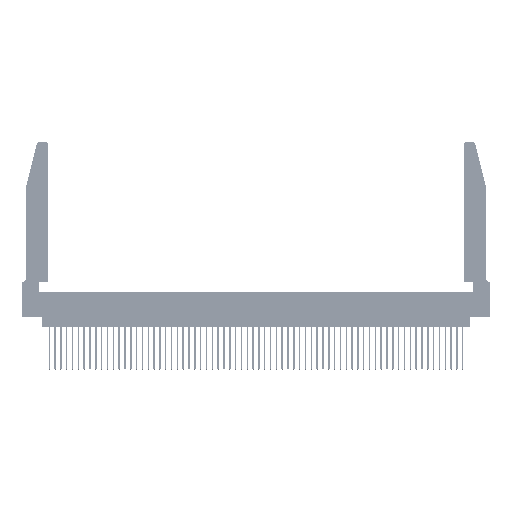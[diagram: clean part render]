
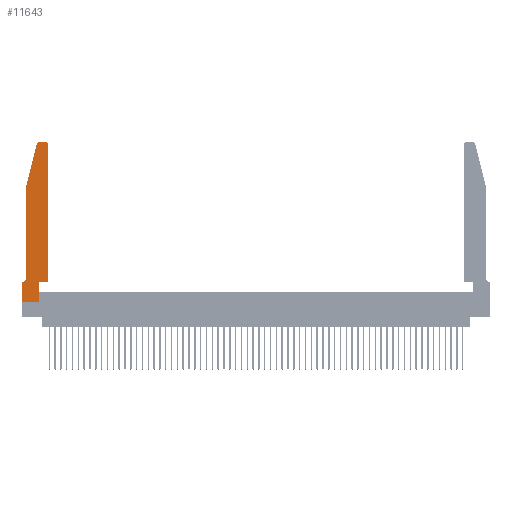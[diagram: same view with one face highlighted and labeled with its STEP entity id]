
A CAD part, top view. The second image highlights one B-rep face of the part: STEP entity #11643.
In plain terms, the highlighted planar face has unit normal (0, 0, 1).
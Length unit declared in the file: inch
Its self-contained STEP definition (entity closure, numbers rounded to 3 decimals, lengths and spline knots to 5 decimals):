
#1697 = CARTESIAN_POINT ( 'NONE',  ( 0.2865, 0., 0.37 ) ) ;
#2220 = CARTESIAN_POINT ( 'NONE',  ( 0.284, 2.72, 0.37 ) ) ;
#2479 = DIRECTION ( 'NONE',  ( 1., 0., 0. ) ) ;
#2614 = ORIENTED_EDGE ( 'NONE', *, *, #24294, .T. ) ;
#3371 = VERTEX_POINT ( 'NONE', #28870 ) ;
#3982 = VECTOR ( 'NONE', #50351, 39.37008 ) ;
#4497 = CARTESIAN_POINT ( 'NONE',  ( 0.2865, 0.35, 0.37 ) ) ;
#6109 = DIRECTION ( 'NONE',  ( 0., 0., -1. ) ) ;
#6855 = VERTEX_POINT ( 'NONE', #46864 ) ;
#7852 = ORIENTED_EDGE ( 'NONE', *, *, #39142, .T. ) ;
#8134 = CARTESIAN_POINT ( 'NONE',  ( 0.4205, 2.72, 0.37 ) ) ;
#8221 = VECTOR ( 'NONE', #50771, 39.37008 ) ;
#9159 = ORIENTED_EDGE ( 'NONE', *, *, #27788, .T. ) ;
#9622 = LINE ( 'NONE', #38343, #36553 ) ;
#9731 = CARTESIAN_POINT ( 'NONE',  ( 0.4205, 2.75, 0.37 ) ) ;
#10589 = DIRECTION ( 'NONE',  ( 1., 0., 0. ) ) ;
#10696 = VECTOR ( 'NONE', #14450, 39.37008 ) ;
#11239 = VERTEX_POINT ( 'NONE', #39124 ) ;
#11420 = VECTOR ( 'NONE', #52880, 39.37008 ) ;
#11643 = ADVANCED_FACE ( 'NONE', ( #20713 ), #40673, .T. ) ;
#12100 = VERTEX_POINT ( 'NONE', #16924 ) ;
#12194 = VERTEX_POINT ( 'NONE', #21421 ) ;
#12627 = DIRECTION ( 'NONE',  ( 1., 0., 0. ) ) ;
#14081 = CARTESIAN_POINT ( 'NONE',  ( 0., 0.35, 0.37 ) ) ;
#14450 = DIRECTION ( 'NONE',  ( 0., -1., 0. ) ) ;
#14970 = CARTESIAN_POINT ( 'NONE',  ( 0.0755, 0.35, 0.37 ) ) ;
#15146 = LINE ( 'NONE', #14970, #8221 ) ;
#16924 = CARTESIAN_POINT ( 'NONE',  ( 0.4505, 0.35, 0.37 ) ) ;
#16975 = CARTESIAN_POINT ( 'NONE',  ( 0., 0., 0.37 ) ) ;
#19117 = ORIENTED_EDGE ( 'NONE', *, *, #36698, .T. ) ;
#19541 = DIRECTION ( 'NONE',  ( -1., 0., 0. ) ) ;
#19923 = DIRECTION ( 'NONE',  ( 0., 0., 1. ) ) ;
#20278 = ORIENTED_EDGE ( 'NONE', *, *, #35598, .T. ) ;
#20713 = FACE_OUTER_BOUND ( 'NONE', #46127, .T. ) ;
#21421 = CARTESIAN_POINT ( 'NONE',  ( 0.0755, 2., 0.37 ) ) ;
#21674 = VERTEX_POINT ( 'NONE', #1697 ) ;
#22527 = LINE ( 'NONE', #23215, #10696 ) ;
#22592 = LINE ( 'NONE', #35314, #11420 ) ;
#23215 = CARTESIAN_POINT ( 'NONE',  ( 0.0755, 2., 0.37 ) ) ;
#23822 = ORIENTED_EDGE ( 'NONE', *, *, #24230, .T. ) ;
#23904 = VECTOR ( 'NONE', #30168, 39.37008 ) ;
#24215 = EDGE_CURVE ( 'NONE', #12194, #3371, #22527, .T. ) ;
#24230 = EDGE_CURVE ( 'NONE', #6855, #32855, #54996, .T. ) ;
#24294 = EDGE_CURVE ( 'NONE', #54954, #6855, #37000, .T. ) ;
#27005 = CARTESIAN_POINT ( 'NONE',  ( 0., 0.35, 0.37 ) ) ;
#27399 = CARTESIAN_POINT ( 'NONE',  ( 0., 0., 0.37 ) ) ;
#27788 = EDGE_CURVE ( 'NONE', #11239, #55626, #15146, .T. ) ;
#27844 = AXIS2_PLACEMENT_3D ( 'NONE', #8134, #39172, #12627 ) ;
#28870 = CARTESIAN_POINT ( 'NONE',  ( 0.0755, 0.42, 0.37 ) ) ;
#29643 = AXIS2_PLACEMENT_3D ( 'NONE', #14081, #35996, #40478 ) ;
#29696 = ORIENTED_EDGE ( 'NONE', *, *, #30423, .T. ) ;
#30034 = EDGE_CURVE ( 'NONE', #12100, #52534, #22592, .T. ) ;
#30168 = DIRECTION ( 'NONE',  ( 1., 0., 0. ) ) ;
#30423 = EDGE_CURVE ( 'NONE', #40318, #21674, #42607, .T. ) ;
#31288 = VERTEX_POINT ( 'NONE', #4497 ) ;
#31449 = DIRECTION ( 'NONE',  ( -0.239, -0.971, 0. ) ) ;
#32543 = DIRECTION ( 'NONE',  ( -1., 0., 0. ) ) ;
#32855 = VERTEX_POINT ( 'NONE', #50223 ) ;
#33283 = LINE ( 'NONE', #27399, #42983 ) ;
#33807 = CIRCLE ( 'NONE', #27844, 0.03 ) ;
#35314 = CARTESIAN_POINT ( 'NONE',  ( 0.4505, 0.35, 0.37 ) ) ;
#35363 = DIRECTION ( 'NONE',  ( 0., -1., 0. ) ) ;
#35598 = EDGE_CURVE ( 'NONE', #32855, #12194, #38312, .T. ) ;
#35996 = DIRECTION ( 'NONE',  ( 0., 0., 1. ) ) ;
#36553 = VECTOR ( 'NONE', #2479, 39.37008 ) ;
#36698 = EDGE_CURVE ( 'NONE', #55626, #40318, #33283, .T. ) ;
#37000 = LINE ( 'NONE', #46197, #50124 ) ;
#37211 = CARTESIAN_POINT ( 'NONE',  ( 0.2865, 0.35, 0.37 ) ) ;
#38312 = LINE ( 'NONE', #54004, #43154 ) ;
#38343 = CARTESIAN_POINT ( 'NONE',  ( 0.4505, 0.35, 0.37 ) ) ;
#39095 = ORIENTED_EDGE ( 'NONE', *, *, #30034, .T. ) ;
#39124 = CARTESIAN_POINT ( 'NONE',  ( 0.0055, 0.35, 0.37 ) ) ;
#39142 = EDGE_CURVE ( 'NONE', #52534, #54954, #33807, .T. ) ;
#39172 = DIRECTION ( 'NONE',  ( 0., 0., 1. ) ) ;
#39556 = CARTESIAN_POINT ( 'NONE',  ( 0., 0., 0.37 ) ) ;
#40318 = VERTEX_POINT ( 'NONE', #39556 ) ;
#40478 = DIRECTION ( 'NONE',  ( 1., 0., 0. ) ) ;
#40673 = PLANE ( 'NONE',  #29643 ) ;
#42216 = CARTESIAN_POINT ( 'NONE',  ( 0.4505, 2.72, 0.37 ) ) ;
#42607 = LINE ( 'NONE', #16975, #23904 ) ;
#42983 = VECTOR ( 'NONE', #35363, 39.37008 ) ;
#43154 = VECTOR ( 'NONE', #31449, 39.37008 ) ;
#43193 = CIRCLE ( 'NONE', #52277, 0.07 ) ;
#44744 = ORIENTED_EDGE ( 'NONE', *, *, #49522, .T. ) ;
#45987 = EDGE_CURVE ( 'NONE', #21674, #31288, #49110, .T. ) ;
#45996 = ORIENTED_EDGE ( 'NONE', *, *, #45987, .T. ) ;
#46127 = EDGE_LOOP ( 'NONE', ( #2614, #23822, #20278, #52236, #44744, #9159, #19117, #29696, #45996, #53489, #39095, #7852 ) ) ;
#46164 = EDGE_CURVE ( 'NONE', #31288, #12100, #9622, .T. ) ;
#46197 = CARTESIAN_POINT ( 'NONE',  ( 0.2605, 2.75, 0.37 ) ) ;
#46864 = CARTESIAN_POINT ( 'NONE',  ( 0.284, 2.75, 0.37 ) ) ;
#49110 = LINE ( 'NONE', #37211, #3982 ) ;
#49522 = EDGE_CURVE ( 'NONE', #3371, #11239, #43193, .T. ) ;
#50124 = VECTOR ( 'NONE', #19541, 39.37008 ) ;
#50223 = CARTESIAN_POINT ( 'NONE',  ( 0.25487, 2.72718, 0.37 ) ) ;
#50351 = DIRECTION ( 'NONE',  ( 0., 1., 0. ) ) ;
#50771 = DIRECTION ( 'NONE',  ( -1., 0., 0. ) ) ;
#52225 = AXIS2_PLACEMENT_3D ( 'NONE', #2220, #19923, #10589 ) ;
#52236 = ORIENTED_EDGE ( 'NONE', *, *, #24215, .T. ) ;
#52277 = AXIS2_PLACEMENT_3D ( 'NONE', #54530, #6109, #32543 ) ;
#52534 = VERTEX_POINT ( 'NONE', #42216 ) ;
#52880 = DIRECTION ( 'NONE',  ( 0., 1., 0. ) ) ;
#53489 = ORIENTED_EDGE ( 'NONE', *, *, #46164, .T. ) ;
#54004 = CARTESIAN_POINT ( 'NONE',  ( 0.0755, 2., 0.37 ) ) ;
#54530 = CARTESIAN_POINT ( 'NONE',  ( 0.0055, 0.42, 0.37 ) ) ;
#54954 = VERTEX_POINT ( 'NONE', #9731 ) ;
#54996 = CIRCLE ( 'NONE', #52225, 0.03 ) ;
#55626 = VERTEX_POINT ( 'NONE', #27005 ) ;
